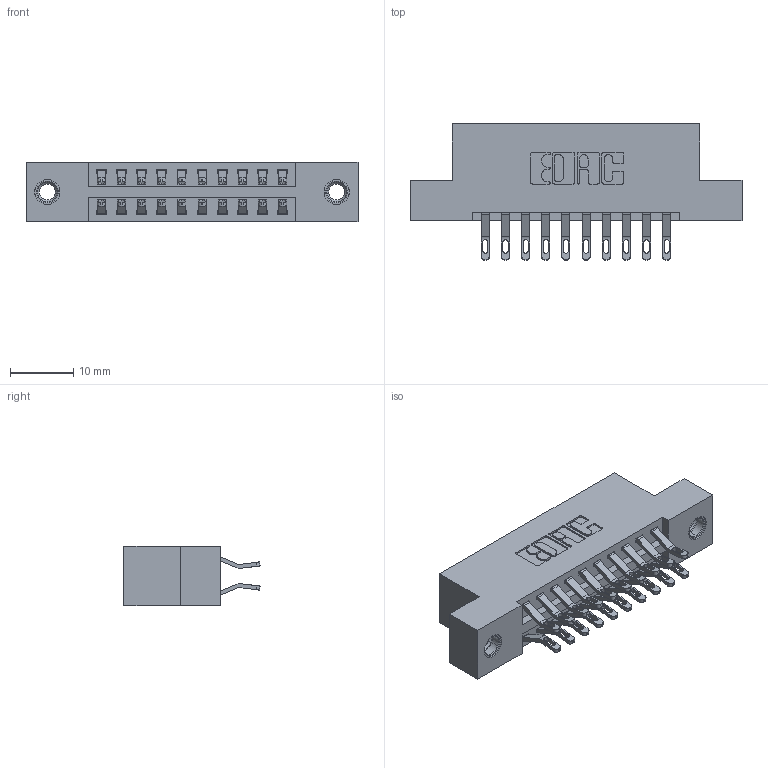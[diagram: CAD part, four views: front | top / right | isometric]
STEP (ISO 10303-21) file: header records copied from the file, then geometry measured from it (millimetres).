
FILE_DESCRIPTION (( 'STEP AP203' ), '1' );
FILE_NAME ('396-020-555-207.STEP', '2019-10-30T03:27:56', ( '' ), ( '' ), 'SwSTEP 2.0', 'SolidWorks 2016', '' );
FILE_SCHEMA (( 'CONFIG_CONTROL_DESIGN' ));
Length unit declared in the file: inch
Products named in the file (4): 396-020-555-207; 346 Part_Flush Mounting Lugs - 0.156 Dia-TI; 345-250-001_345-250-005-103; 345-292-001_555 Tail
Assembly tree (23 placements, depth 2):
  396-020-555-207
    346 Part_Flush Mounting Lugs - 0.156 Dia-TI
    345-292-001_555 Tail  x20
    345-250-001_345-250-005-103  x2
Bounding box: 52.32 x 21.46 x 9.4 mm (x, y, z)
Volume: 4898.2 mm3; surface area: 6470.5 mm2
Topology: 23 solids, 23 shells, 1342 faces, 4125 edges, 2742 vertices
Faces by surface type: plane 768, cylinder 558, cone 12, torus 4
Entity records: 12346 total; most frequent: CARTESIAN_POINT 2097, ORIENTED_EDGE 1994, DIRECTION 1895, EDGE_CURVE 997, LINE 785, VECTOR 785, VERTEX_POINT 660, AXIS2_PLACEMENT_3D 555
